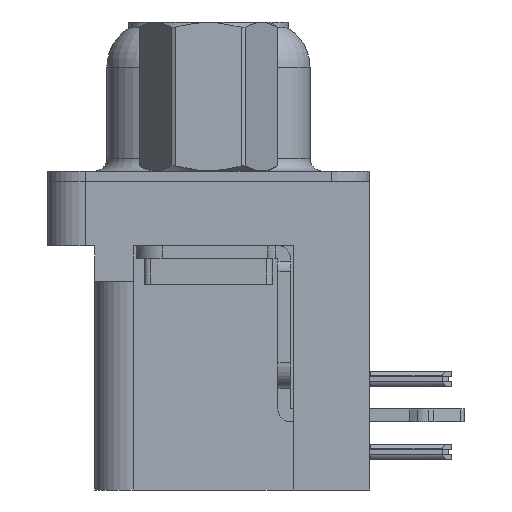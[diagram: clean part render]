
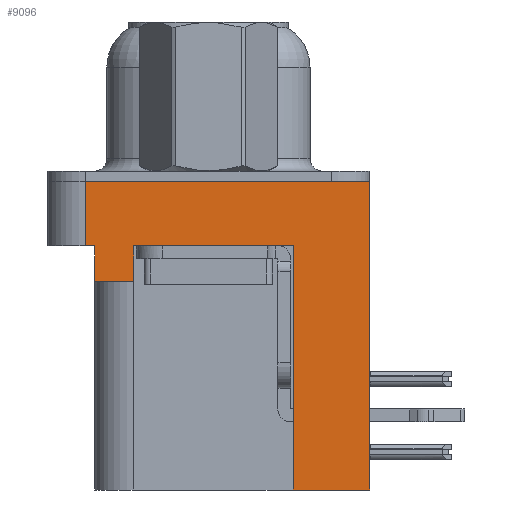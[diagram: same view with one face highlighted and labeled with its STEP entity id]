
A CAD part, left-side view. The second image highlights one B-rep face of the part: STEP entity #9096.
In plain terms, the highlighted planar face has unit normal (-1, 0, 0).
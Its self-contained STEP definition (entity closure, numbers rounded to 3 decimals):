
#329 = ORIENTED_EDGE ( 'NONE', *, *, #34745, .T. ) ;
#383 = EDGE_CURVE ( 'NONE', #37473, #38449, #32090, .T. ) ;
#1721 = ORIENTED_EDGE ( 'NONE', *, *, #22865, .F. ) ;
#2045 = LINE ( 'NONE', #23190, #30542 ) ;
#2712 = DIRECTION ( 'NONE',  ( 0., 0., 1. ) ) ;
#2991 = DIRECTION ( 'NONE',  ( 0., 0., 1. ) ) ;
#3374 = EDGE_CURVE ( 'NONE', #23444, #12684, #20844, .T. ) ;
#3807 = DIRECTION ( 'NONE',  ( 0., 1., 0. ) ) ;
#5467 = CARTESIAN_POINT ( 'NONE',  ( -2.91, -3.295, -2.5 ) ) ;
#6169 = CARTESIAN_POINT ( 'NONE',  ( -2.91, 4.775, -2.5 ) ) ;
#6782 = EDGE_CURVE ( 'NONE', #38449, #30141, #10607, .T. ) ;
#7041 = LINE ( 'NONE', #40883, #23041 ) ;
#8605 = CARTESIAN_POINT ( 'NONE',  ( -2.91, 4.425, -2.5 ) ) ;
#8669 = VECTOR ( 'NONE', #8940, 1000. ) ;
#8728 = CARTESIAN_POINT ( 'NONE',  ( -2.91, -6.275, -2.5 ) ) ;
#8809 = CARTESIAN_POINT ( 'NONE',  ( -2.91, 2.895, -3.9 ) ) ;
#8894 = EDGE_CURVE ( 'NONE', #37473, #12684, #34703, .T. ) ;
#8940 = DIRECTION ( 'NONE',  ( 0., 0., 1. ) ) ;
#9096 = ADVANCED_FACE ( 'NONE', ( #36177 ), #34120, .T. ) ;
#9218 = CARTESIAN_POINT ( 'NONE',  ( -2.91, 4.775, 0. ) ) ;
#9316 = EDGE_CURVE ( 'NONE', #13556, #25472, #36143, .T. ) ;
#9530 = CARTESIAN_POINT ( 'NONE',  ( -2.91, -6.275, -12. ) ) ;
#9714 = ORIENTED_EDGE ( 'NONE', *, *, #9316, .T. ) ;
#10607 = LINE ( 'NONE', #27821, #35004 ) ;
#11926 = CARTESIAN_POINT ( 'NONE',  ( -2.91, 2.895, -3.9 ) ) ;
#11931 = ORIENTED_EDGE ( 'NONE', *, *, #12910, .F. ) ;
#12661 = DIRECTION ( 'NONE',  ( 0., -1., 0. ) ) ;
#12684 = VERTEX_POINT ( 'NONE', #20687 ) ;
#12711 = LINE ( 'NONE', #19805, #28112 ) ;
#12910 = EDGE_CURVE ( 'NONE', #26014, #23444, #16169, .T. ) ;
#13556 = VERTEX_POINT ( 'NONE', #11926 ) ;
#14148 = CARTESIAN_POINT ( 'NONE',  ( -2.91, -3.295, -12. ) ) ;
#14674 = VECTOR ( 'NONE', #3807, 1000. ) ;
#15508 = CARTESIAN_POINT ( 'NONE',  ( -2.91, 2.895, -2.5 ) ) ;
#15980 = DIRECTION ( 'NONE',  ( -1., 0., 0. ) ) ;
#16169 = LINE ( 'NONE', #25633, #32674 ) ;
#16877 = DIRECTION ( 'NONE',  ( 0., 0., 1. ) ) ;
#17241 = DIRECTION ( 'NONE',  ( 0., -1., 0. ) ) ;
#17957 = ORIENTED_EDGE ( 'NONE', *, *, #3374, .F. ) ;
#18347 = EDGE_CURVE ( 'NONE', #25472, #30141, #7041, .T. ) ;
#18589 = EDGE_CURVE ( 'NONE', #23056, #22395, #2045, .T. ) ;
#18932 = CARTESIAN_POINT ( 'NONE',  ( -2.91, -6.275, -2.5 ) ) ;
#19311 = ORIENTED_EDGE ( 'NONE', *, *, #8894, .T. ) ;
#19596 = DIRECTION ( 'NONE',  ( 0., 0., 1. ) ) ;
#19805 = CARTESIAN_POINT ( 'NONE',  ( -2.91, 4.425, -3.9 ) ) ;
#20415 = CARTESIAN_POINT ( 'NONE',  ( -2.91, 4.425, -3.9 ) ) ;
#20687 = CARTESIAN_POINT ( 'NONE',  ( -2.91, -6.275, 0. ) ) ;
#20844 = LINE ( 'NONE', #33511, #21317 ) ;
#20847 = ORIENTED_EDGE ( 'NONE', *, *, #383, .F. ) ;
#21317 = VECTOR ( 'NONE', #17241, 1000. ) ;
#22379 = DIRECTION ( 'NONE',  ( 0., 0., 1. ) ) ;
#22395 = VERTEX_POINT ( 'NONE', #8605 ) ;
#22865 = EDGE_CURVE ( 'NONE', #13556, #23056, #12711, .T. ) ;
#23041 = VECTOR ( 'NONE', #34494, 1000. ) ;
#23056 = VERTEX_POINT ( 'NONE', #20415 ) ;
#23190 = CARTESIAN_POINT ( 'NONE',  ( -2.91, 4.425, -3.9 ) ) ;
#23237 = VECTOR ( 'NONE', #22379, 1000. ) ;
#23444 = VERTEX_POINT ( 'NONE', #9218 ) ;
#24176 = VECTOR ( 'NONE', #12661, 1000. ) ;
#25472 = VERTEX_POINT ( 'NONE', #15508 ) ;
#25631 = DIRECTION ( 'NONE',  ( 0., 1., 0. ) ) ;
#25633 = CARTESIAN_POINT ( 'NONE',  ( -2.91, 4.775, -2.5 ) ) ;
#26014 = VERTEX_POINT ( 'NONE', #6169 ) ;
#26653 = LINE ( 'NONE', #18932, #24176 ) ;
#27821 = CARTESIAN_POINT ( 'NONE',  ( -2.91, -3.295, -12. ) ) ;
#28112 = VECTOR ( 'NONE', #25631, 1000. ) ;
#28437 = ORIENTED_EDGE ( 'NONE', *, *, #6782, .F. ) ;
#30141 = VERTEX_POINT ( 'NONE', #5467 ) ;
#30542 = VECTOR ( 'NONE', #19596, 1000. ) ;
#32090 = LINE ( 'NONE', #35594, #14674 ) ;
#32478 = ORIENTED_EDGE ( 'NONE', *, *, #18347, .T. ) ;
#32674 = VECTOR ( 'NONE', #16877, 1000. ) ;
#33432 = ORIENTED_EDGE ( 'NONE', *, *, #18589, .F. ) ;
#33511 = CARTESIAN_POINT ( 'NONE',  ( -2.91, -6.275, 0. ) ) ;
#34120 = PLANE ( 'NONE',  #34345 ) ;
#34345 = AXIS2_PLACEMENT_3D ( 'NONE', #8728, #15980, #2991 ) ;
#34494 = DIRECTION ( 'NONE',  ( 0., -1., 0. ) ) ;
#34703 = LINE ( 'NONE', #35571, #23237 ) ;
#34745 = EDGE_CURVE ( 'NONE', #26014, #22395, #26653, .T. ) ;
#35004 = VECTOR ( 'NONE', #2712, 1000. ) ;
#35571 = CARTESIAN_POINT ( 'NONE',  ( -2.91, -6.275, -2.5 ) ) ;
#35594 = CARTESIAN_POINT ( 'NONE',  ( -2.91, -3.295, -12. ) ) ;
#36143 = LINE ( 'NONE', #8809, #8669 ) ;
#36177 = FACE_OUTER_BOUND ( 'NONE', #40461, .T. ) ;
#37473 = VERTEX_POINT ( 'NONE', #9530 ) ;
#38449 = VERTEX_POINT ( 'NONE', #14148 ) ;
#40461 = EDGE_LOOP ( 'NONE', ( #17957, #11931, #329, #33432, #1721, #9714, #32478, #28437, #20847, #19311 ) ) ;
#40883 = CARTESIAN_POINT ( 'NONE',  ( -2.91, -6.275, -2.5 ) ) ;
